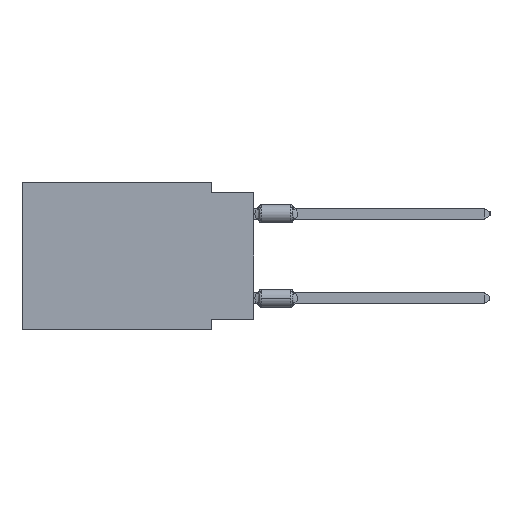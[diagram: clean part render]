
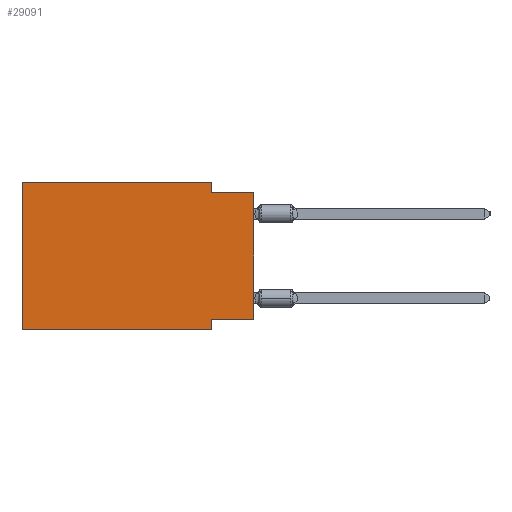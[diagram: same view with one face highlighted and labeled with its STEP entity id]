
A CAD part, left-side view. The second image highlights one B-rep face of the part: STEP entity #29091.
In plain terms, the highlighted planar face has unit normal (-1, 0, 0).
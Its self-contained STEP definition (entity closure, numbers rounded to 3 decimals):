
#85 = VECTOR ( 'NONE', #9389, 1000. ) ;
#265 = CARTESIAN_POINT ( 'NONE',  ( 0., 0., -0.635 ) ) ;
#467 = FACE_OUTER_BOUND ( 'NONE', #23942, .T. ) ;
#1154 = VECTOR ( 'NONE', #25493, 1000. ) ;
#1519 = VECTOR ( 'NONE', #46092, 1000. ) ;
#2224 = EDGE_CURVE ( 'NONE', #23969, #28617, #29035, .T. ) ;
#3271 = DIRECTION ( 'NONE',  ( 0., 0., 1. ) ) ;
#4366 = VECTOR ( 'NONE', #3271, 1000. ) ;
#4930 = CARTESIAN_POINT ( 'NONE',  ( 0., 13.97, 0. ) ) ;
#5141 = DIRECTION ( 'NONE',  ( 0., 0., -1. ) ) ;
#7588 = EDGE_CURVE ( 'NONE', #21810, #9244, #28293, .T. ) ;
#8543 = CARTESIAN_POINT ( 'NONE',  ( 0., 0., -8.255 ) ) ;
#9244 = VERTEX_POINT ( 'NONE', #56274 ) ;
#9389 = DIRECTION ( 'NONE',  ( 0., 1., 0. ) ) ;
#9515 = CARTESIAN_POINT ( 'NONE',  ( 0., 0., -0.635 ) ) ;
#9815 = CARTESIAN_POINT ( 'NONE',  ( 0., 13.97, 0. ) ) ;
#10457 = CARTESIAN_POINT ( 'NONE',  ( 0., 2.54, -8.89 ) ) ;
#12347 = ORIENTED_EDGE ( 'NONE', *, *, #48606, .T. ) ;
#12794 = VECTOR ( 'NONE', #14396, 1000. ) ;
#12872 = CARTESIAN_POINT ( 'NONE',  ( 0., 13.97, -8.89 ) ) ;
#13765 = LINE ( 'NONE', #8543, #85 ) ;
#14396 = DIRECTION ( 'NONE',  ( 0., -1., 0. ) ) ;
#15640 = LINE ( 'NONE', #33475, #41049 ) ;
#15938 = DIRECTION ( 'NONE',  ( 0., 0., -1. ) ) ;
#17159 = CARTESIAN_POINT ( 'NONE',  ( 0., 13.97, -8.89 ) ) ;
#21810 = VERTEX_POINT ( 'NONE', #51676 ) ;
#22367 = VERTEX_POINT ( 'NONE', #50784 ) ;
#22876 = CARTESIAN_POINT ( 'NONE',  ( 0., 13.97, 0. ) ) ;
#23077 = ORIENTED_EDGE ( 'NONE', *, *, #2224, .F. ) ;
#23942 = EDGE_LOOP ( 'NONE', ( #28542, #44400, #33094, #40598, #23077, #12347, #56713, #26693 ) ) ;
#23969 = VERTEX_POINT ( 'NONE', #17159 ) ;
#24172 = CARTESIAN_POINT ( 'NONE',  ( 0., 2.54, 0. ) ) ;
#25493 = DIRECTION ( 'NONE',  ( 0., -1., 0. ) ) ;
#25609 = VERTEX_POINT ( 'NONE', #10457 ) ;
#26305 = AXIS2_PLACEMENT_3D ( 'NONE', #9815, #27677, #5141 ) ;
#26693 = ORIENTED_EDGE ( 'NONE', *, *, #28186, .F. ) ;
#27677 = DIRECTION ( 'NONE',  ( 1., 0., 0. ) ) ;
#27977 = PLANE ( 'NONE',  #26305 ) ;
#28186 = EDGE_CURVE ( 'NONE', #22367, #44159, #13765, .T. ) ;
#28293 = LINE ( 'NONE', #24172, #45001 ) ;
#28542 = ORIENTED_EDGE ( 'NONE', *, *, #33577, .T. ) ;
#28617 = VERTEX_POINT ( 'NONE', #4930 ) ;
#29035 = LINE ( 'NONE', #29614, #4366 ) ;
#29091 = ADVANCED_FACE ( 'NONE', ( #467 ), #27977, .F. ) ;
#29614 = CARTESIAN_POINT ( 'NONE',  ( 0., 13.97, 0. ) ) ;
#33094 = ORIENTED_EDGE ( 'NONE', *, *, #7588, .F. ) ;
#33475 = CARTESIAN_POINT ( 'NONE',  ( 0., 2.54, -8.89 ) ) ;
#33577 = EDGE_CURVE ( 'NONE', #22367, #45842, #35983, .T. ) ;
#35983 = LINE ( 'NONE', #53826, #41712 ) ;
#36368 = EDGE_CURVE ( 'NONE', #44159, #25609, #15640, .T. ) ;
#36434 = LINE ( 'NONE', #9515, #1519 ) ;
#40598 = ORIENTED_EDGE ( 'NONE', *, *, #56375, .F. ) ;
#41049 = VECTOR ( 'NONE', #15938, 1000. ) ;
#41712 = VECTOR ( 'NONE', #45356, 1000. ) ;
#42912 = DIRECTION ( 'NONE',  ( 0., 0., -1. ) ) ;
#43633 = LINE ( 'NONE', #12872, #1154 ) ;
#44159 = VERTEX_POINT ( 'NONE', #48685 ) ;
#44400 = ORIENTED_EDGE ( 'NONE', *, *, #45026, .F. ) ;
#45001 = VECTOR ( 'NONE', #42912, 1000. ) ;
#45026 = EDGE_CURVE ( 'NONE', #9244, #45842, #36434, .T. ) ;
#45356 = DIRECTION ( 'NONE',  ( 0., 0., 1. ) ) ;
#45842 = VERTEX_POINT ( 'NONE', #265 ) ;
#46092 = DIRECTION ( 'NONE',  ( 0., -1., 0. ) ) ;
#48606 = EDGE_CURVE ( 'NONE', #23969, #25609, #43633, .T. ) ;
#48685 = CARTESIAN_POINT ( 'NONE',  ( 0., 2.54, -8.255 ) ) ;
#50784 = CARTESIAN_POINT ( 'NONE',  ( 0., 0., -8.255 ) ) ;
#50972 = LINE ( 'NONE', #22876, #12794 ) ;
#51676 = CARTESIAN_POINT ( 'NONE',  ( 0., 2.54, 0. ) ) ;
#53826 = CARTESIAN_POINT ( 'NONE',  ( 0., 0., 0. ) ) ;
#56274 = CARTESIAN_POINT ( 'NONE',  ( 0., 2.54, -0.635 ) ) ;
#56375 = EDGE_CURVE ( 'NONE', #28617, #21810, #50972, .T. ) ;
#56713 = ORIENTED_EDGE ( 'NONE', *, *, #36368, .F. ) ;
